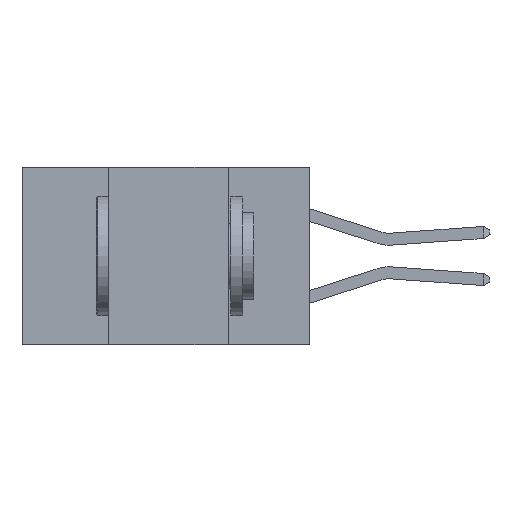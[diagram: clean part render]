
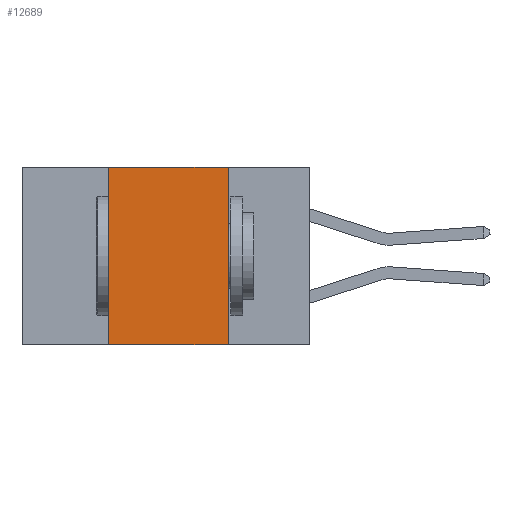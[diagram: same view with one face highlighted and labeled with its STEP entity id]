
A CAD part, left-side view. The second image highlights one B-rep face of the part: STEP entity #12689.
In plain terms, the highlighted planar face has unit normal (-1, 0, 0).
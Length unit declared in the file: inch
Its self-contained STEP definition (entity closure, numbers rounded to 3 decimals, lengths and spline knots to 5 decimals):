
#514 = VECTOR ( 'NONE', #4826, 39.37008 ) ;
#608 = LINE ( 'NONE', #9779, #12791 ) ;
#895 = PLANE ( 'NONE',  #11258 ) ;
#949 = CARTESIAN_POINT ( 'NONE',  ( 0., 0.6, -0.37 ) ) ;
#1315 = CARTESIAN_POINT ( 'NONE',  ( 0., 0.17, 0. ) ) ;
#1483 = EDGE_CURVE ( 'NONE', #14913, #10709, #5519, .T. ) ;
#1658 = DIRECTION ( 'NONE',  ( 0., 0., 1. ) ) ;
#3423 = FACE_OUTER_BOUND ( 'NONE', #12836, .T. ) ;
#4763 = EDGE_CURVE ( 'NONE', #14913, #6873, #12508, .T. ) ;
#4826 = DIRECTION ( 'NONE',  ( 0., -1., 0. ) ) ;
#5519 = LINE ( 'NONE', #8144, #13261 ) ;
#5766 = VECTOR ( 'NONE', #10086, 39.37008 ) ;
#5894 = DIRECTION ( 'NONE',  ( 0., -1., 0. ) ) ;
#6028 = CARTESIAN_POINT ( 'NONE',  ( 0., 0.6, 0. ) ) ;
#6220 = LINE ( 'NONE', #8640, #5766 ) ;
#6287 = EDGE_CURVE ( 'NONE', #10709, #8882, #608, .T. ) ;
#6873 = VERTEX_POINT ( 'NONE', #12381 ) ;
#8144 = CARTESIAN_POINT ( 'NONE',  ( 0., 0.42, -0.37 ) ) ;
#8285 = EDGE_CURVE ( 'NONE', #8882, #6873, #6220, .T. ) ;
#8640 = CARTESIAN_POINT ( 'NONE',  ( 0., 0.17, -0.37 ) ) ;
#8882 = VERTEX_POINT ( 'NONE', #1315 ) ;
#9452 = ORIENTED_EDGE ( 'NONE', *, *, #1483, .F. ) ;
#9779 = CARTESIAN_POINT ( 'NONE',  ( 0., 0.6, 0. ) ) ;
#10086 = DIRECTION ( 'NONE',  ( 0., 0., -1. ) ) ;
#10340 = ORIENTED_EDGE ( 'NONE', *, *, #6287, .F. ) ;
#10385 = CARTESIAN_POINT ( 'NONE',  ( 0., 0.42, -0.37 ) ) ;
#10709 = VERTEX_POINT ( 'NONE', #12474 ) ;
#11175 = DIRECTION ( 'NONE',  ( 1., 0., 0. ) ) ;
#11258 = AXIS2_PLACEMENT_3D ( 'NONE', #6028, #11175, #16301 ) ;
#12381 = CARTESIAN_POINT ( 'NONE',  ( 0., 0.17, -0.37 ) ) ;
#12474 = CARTESIAN_POINT ( 'NONE',  ( 0., 0.42, 0. ) ) ;
#12508 = LINE ( 'NONE', #949, #514 ) ;
#12689 = ADVANCED_FACE ( 'NONE', ( #3423 ), #895, .F. ) ;
#12791 = VECTOR ( 'NONE', #5894, 39.37008 ) ;
#12836 = EDGE_LOOP ( 'NONE', ( #13210, #10340, #9452, #13290 ) ) ;
#13210 = ORIENTED_EDGE ( 'NONE', *, *, #8285, .F. ) ;
#13261 = VECTOR ( 'NONE', #1658, 39.37008 ) ;
#13290 = ORIENTED_EDGE ( 'NONE', *, *, #4763, .T. ) ;
#14913 = VERTEX_POINT ( 'NONE', #10385 ) ;
#16301 = DIRECTION ( 'NONE',  ( 0., 0., -1. ) ) ;
